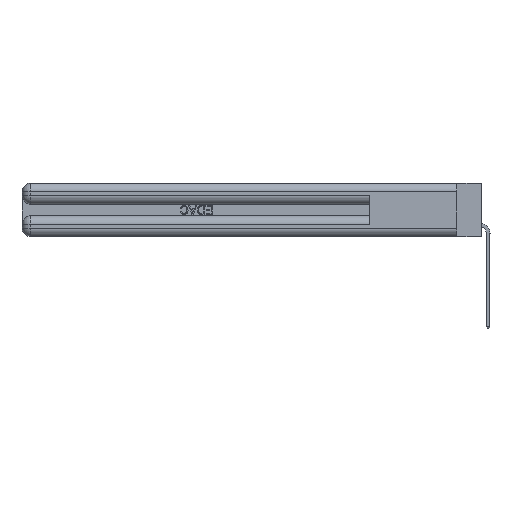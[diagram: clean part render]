
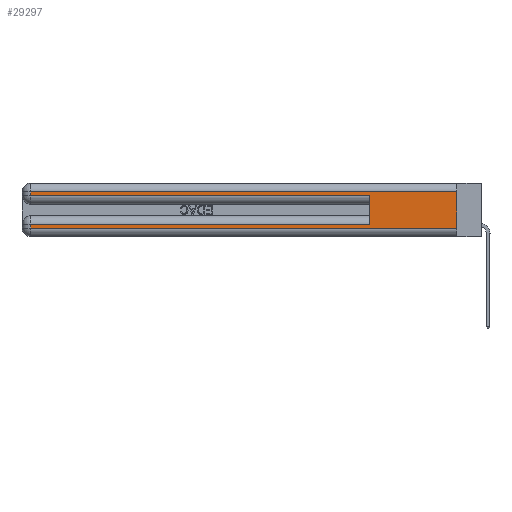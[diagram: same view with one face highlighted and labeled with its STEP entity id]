
A CAD part, left-side view. The second image highlights one B-rep face of the part: STEP entity #29297.
In plain terms, the highlighted planar face has unit normal (-1, 0, 0).
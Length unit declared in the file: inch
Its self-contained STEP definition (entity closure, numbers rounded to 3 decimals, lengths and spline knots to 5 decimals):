
#207 = EDGE_CURVE ( 'NONE', #13852, #7746, #33512, .T. ) ;
#250 = VECTOR ( 'NONE', #4310, 39.37008 ) ;
#859 = EDGE_CURVE ( 'NONE', #9386, #13852, #13689, .T. ) ;
#1366 = VERTEX_POINT ( 'NONE', #27287 ) ;
#1662 = ORIENTED_EDGE ( 'NONE', *, *, #29368, .T. ) ;
#2091 = VECTOR ( 'NONE', #5783, 39.37008 ) ;
#3406 = ORIENTED_EDGE ( 'NONE', *, *, #21302, .F. ) ;
#3811 = DIRECTION ( 'NONE',  ( 0., 1., 0. ) ) ;
#4301 = FACE_OUTER_BOUND ( 'NONE', #9457, .T. ) ;
#4310 = DIRECTION ( 'NONE',  ( 0., 0., -1. ) ) ;
#5751 = ORIENTED_EDGE ( 'NONE', *, *, #12853, .T. ) ;
#5783 = DIRECTION ( 'NONE',  ( 0., -1., 0. ) ) ;
#6100 = DIRECTION ( 'NONE',  ( 0., 1., 0. ) ) ;
#6425 = PLANE ( 'NONE',  #8272 ) ;
#7517 = VECTOR ( 'NONE', #9907, 39.37008 ) ;
#7746 = VERTEX_POINT ( 'NONE', #11135 ) ;
#8029 = LINE ( 'NONE', #11808, #2091 ) ;
#8272 = AXIS2_PLACEMENT_3D ( 'NONE', #9323, #24210, #36706 ) ;
#9323 = CARTESIAN_POINT ( 'NONE',  ( 0., 0., 0.37 ) ) ;
#9386 = VERTEX_POINT ( 'NONE', #10961 ) ;
#9457 = EDGE_LOOP ( 'NONE', ( #17365, #31718, #17867, #43757, #3406, #5751, #1662, #36354 ) ) ;
#9784 = DIRECTION ( 'NONE',  ( 0., 0., -1. ) ) ;
#9907 = DIRECTION ( 'NONE',  ( 0., 0., 1. ) ) ;
#10116 = CARTESIAN_POINT ( 'NONE',  ( 0., 2.94, 0.085 ) ) ;
#10476 = VERTEX_POINT ( 'NONE', #10116 ) ;
#10961 = CARTESIAN_POINT ( 'NONE',  ( 0., 2.94, 0.31 ) ) ;
#11135 = CARTESIAN_POINT ( 'NONE',  ( 0., 0.6, 0.285 ) ) ;
#11617 = LINE ( 'NONE', #37933, #29255 ) ;
#11808 = CARTESIAN_POINT ( 'NONE',  ( 0., 0., 0.06 ) ) ;
#12715 = CARTESIAN_POINT ( 'NONE',  ( 0., 0., 0.31 ) ) ;
#12853 = EDGE_CURVE ( 'NONE', #43826, #10476, #16249, .T. ) ;
#12902 = CARTESIAN_POINT ( 'NONE',  ( 0., 2.94, 0.37 ) ) ;
#13689 = LINE ( 'NONE', #28279, #250 ) ;
#13852 = VERTEX_POINT ( 'NONE', #18204 ) ;
#15250 = VERTEX_POINT ( 'NONE', #23403 ) ;
#16249 = LINE ( 'NONE', #17159, #42523 ) ;
#17159 = CARTESIAN_POINT ( 'NONE',  ( 0., 0., 0.085 ) ) ;
#17365 = ORIENTED_EDGE ( 'NONE', *, *, #38887, .F. ) ;
#17438 = VECTOR ( 'NONE', #6100, 39.37008 ) ;
#17465 = EDGE_CURVE ( 'NONE', #35569, #9386, #36770, .T. ) ;
#17867 = ORIENTED_EDGE ( 'NONE', *, *, #859, .T. ) ;
#18204 = CARTESIAN_POINT ( 'NONE',  ( 0., 2.94, 0.285 ) ) ;
#19523 = CARTESIAN_POINT ( 'NONE',  ( 0., 0., 0.285 ) ) ;
#19962 = DIRECTION ( 'NONE',  ( 0., -1., 0. ) ) ;
#21302 = EDGE_CURVE ( 'NONE', #43826, #7746, #21413, .T. ) ;
#21413 = LINE ( 'NONE', #26911, #7517 ) ;
#22542 = VECTOR ( 'NONE', #9784, 39.37008 ) ;
#23403 = CARTESIAN_POINT ( 'NONE',  ( 0., 2.94, 0.06 ) ) ;
#24142 = CARTESIAN_POINT ( 'NONE',  ( 0., 0.6, 0.085 ) ) ;
#24210 = DIRECTION ( 'NONE',  ( 1., 0., 0. ) ) ;
#26911 = CARTESIAN_POINT ( 'NONE',  ( 0., 0.6, 0.145 ) ) ;
#27287 = CARTESIAN_POINT ( 'NONE',  ( 0., 0., 0.06 ) ) ;
#28279 = CARTESIAN_POINT ( 'NONE',  ( 0., 2.94, 0.37 ) ) ;
#28703 = VECTOR ( 'NONE', #19962, 39.37008 ) ;
#29255 = VECTOR ( 'NONE', #34329, 39.37008 ) ;
#29297 = ADVANCED_FACE ( 'NONE', ( #4301 ), #6425, .F. ) ;
#29368 = EDGE_CURVE ( 'NONE', #10476, #15250, #38653, .T. ) ;
#31718 = ORIENTED_EDGE ( 'NONE', *, *, #17465, .T. ) ;
#33512 = LINE ( 'NONE', #19523, #28703 ) ;
#34329 = DIRECTION ( 'NONE',  ( 0., 0., -1. ) ) ;
#35569 = VERTEX_POINT ( 'NONE', #39601 ) ;
#36354 = ORIENTED_EDGE ( 'NONE', *, *, #43495, .T. ) ;
#36706 = DIRECTION ( 'NONE',  ( 0., 0., -1. ) ) ;
#36770 = LINE ( 'NONE', #12715, #17438 ) ;
#37933 = CARTESIAN_POINT ( 'NONE',  ( 0., 0., 0.37 ) ) ;
#38653 = LINE ( 'NONE', #12902, #22542 ) ;
#38887 = EDGE_CURVE ( 'NONE', #35569, #1366, #11617, .T. ) ;
#39601 = CARTESIAN_POINT ( 'NONE',  ( 0., 0., 0.31 ) ) ;
#42523 = VECTOR ( 'NONE', #3811, 39.37008 ) ;
#43495 = EDGE_CURVE ( 'NONE', #15250, #1366, #8029, .T. ) ;
#43757 = ORIENTED_EDGE ( 'NONE', *, *, #207, .T. ) ;
#43826 = VERTEX_POINT ( 'NONE', #24142 ) ;
